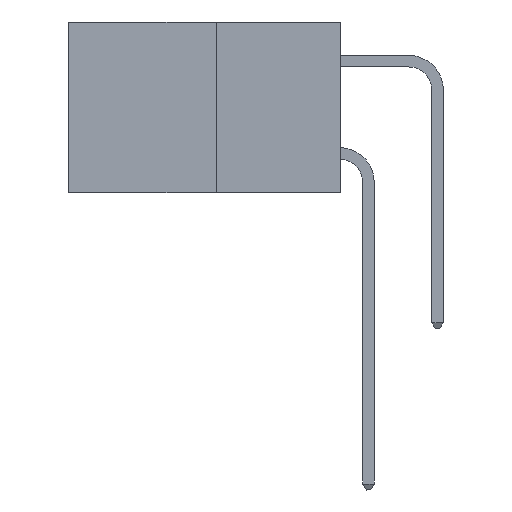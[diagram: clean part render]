
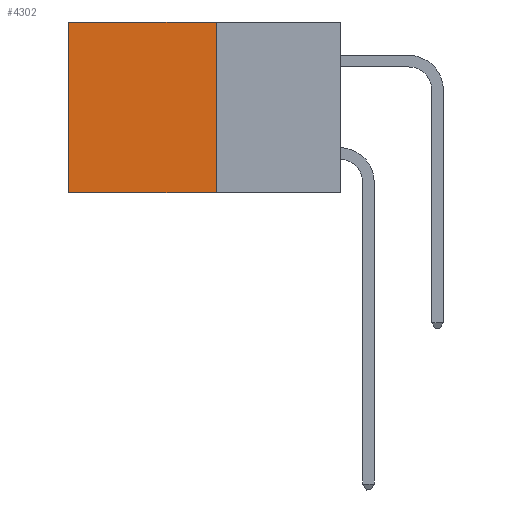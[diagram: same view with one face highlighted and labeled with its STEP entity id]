
A CAD part, left-side view. The second image highlights one B-rep face of the part: STEP entity #4302.
In plain terms, the highlighted planar face has unit normal (-1, 0, 0).
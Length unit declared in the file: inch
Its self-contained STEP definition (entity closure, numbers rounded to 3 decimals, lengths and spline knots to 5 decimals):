
#869 = DIRECTION ( 'NONE',  ( 0., 0., -1. ) ) ;
#2353 = DIRECTION ( 'NONE',  ( 0., 0., -1. ) ) ;
#4006 = LINE ( 'NONE', #4125, #12766 ) ;
#4125 = CARTESIAN_POINT ( 'NONE',  ( 0.277, 0.27, -0.37 ) ) ;
#4302 = ADVANCED_FACE ( 'NONE', ( #21251 ), #18252, .F. ) ;
#4497 = VECTOR ( 'NONE', #19251, 39.37008 ) ;
#4537 = VECTOR ( 'NONE', #11944, 39.37008 ) ;
#4705 = VERTEX_POINT ( 'NONE', #8854 ) ;
#5004 = CARTESIAN_POINT ( 'NONE',  ( 0.277, 0.27, -0.37 ) ) ;
#6188 = EDGE_CURVE ( 'NONE', #4705, #8404, #4006, .T. ) ;
#6790 = DIRECTION ( 'NONE',  ( 0., 1., 0. ) ) ;
#7144 = ORIENTED_EDGE ( 'NONE', *, *, #13166, .T. ) ;
#7152 = VECTOR ( 'NONE', #6790, 39.37008 ) ;
#8136 = VERTEX_POINT ( 'NONE', #14019 ) ;
#8300 = EDGE_LOOP ( 'NONE', ( #7144, #11219, #13385, #13488 ) ) ;
#8404 = VERTEX_POINT ( 'NONE', #9516 ) ;
#8854 = CARTESIAN_POINT ( 'NONE',  ( 0.277, 0.27, 0. ) ) ;
#9144 = LINE ( 'NONE', #20886, #4497 ) ;
#9328 = LINE ( 'NONE', #11971, #7152 ) ;
#9516 = CARTESIAN_POINT ( 'NONE',  ( 0.277, 0.27, -0.37 ) ) ;
#10833 = VERTEX_POINT ( 'NONE', #13361 ) ;
#11219 = ORIENTED_EDGE ( 'NONE', *, *, #12276, .F. ) ;
#11341 = AXIS2_PLACEMENT_3D ( 'NONE', #19990, #11368, #869 ) ;
#11368 = DIRECTION ( 'NONE',  ( 1., 0., 0. ) ) ;
#11944 = DIRECTION ( 'NONE',  ( 0., 1., 0. ) ) ;
#11971 = CARTESIAN_POINT ( 'NONE',  ( 0.277, 0.27, 0. ) ) ;
#12276 = EDGE_CURVE ( 'NONE', #8404, #8136, #22428, .T. ) ;
#12766 = VECTOR ( 'NONE', #2353, 39.37008 ) ;
#13166 = EDGE_CURVE ( 'NONE', #10833, #8136, #9144, .T. ) ;
#13361 = CARTESIAN_POINT ( 'NONE',  ( 0.277, 0.59, 0. ) ) ;
#13385 = ORIENTED_EDGE ( 'NONE', *, *, #6188, .F. ) ;
#13488 = ORIENTED_EDGE ( 'NONE', *, *, #15985, .T. ) ;
#14019 = CARTESIAN_POINT ( 'NONE',  ( 0.277, 0.59, -0.37 ) ) ;
#15985 = EDGE_CURVE ( 'NONE', #4705, #10833, #9328, .T. ) ;
#18252 = PLANE ( 'NONE',  #11341 ) ;
#19251 = DIRECTION ( 'NONE',  ( 0., 0., -1. ) ) ;
#19990 = CARTESIAN_POINT ( 'NONE',  ( 0.277, 0.27, -0.37 ) ) ;
#20886 = CARTESIAN_POINT ( 'NONE',  ( 0.277, 0.59, -0.37 ) ) ;
#21251 = FACE_OUTER_BOUND ( 'NONE', #8300, .T. ) ;
#22428 = LINE ( 'NONE', #5004, #4537 ) ;
